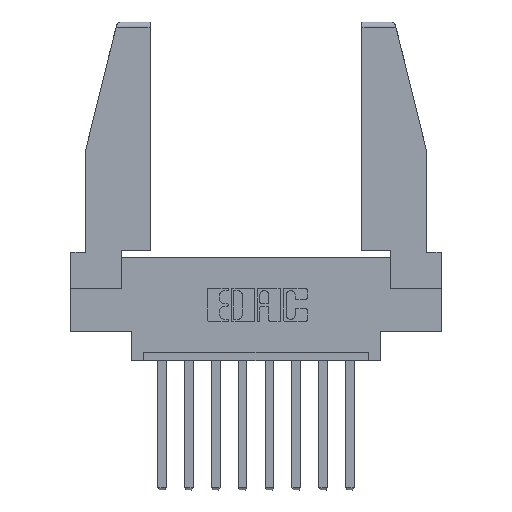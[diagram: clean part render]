
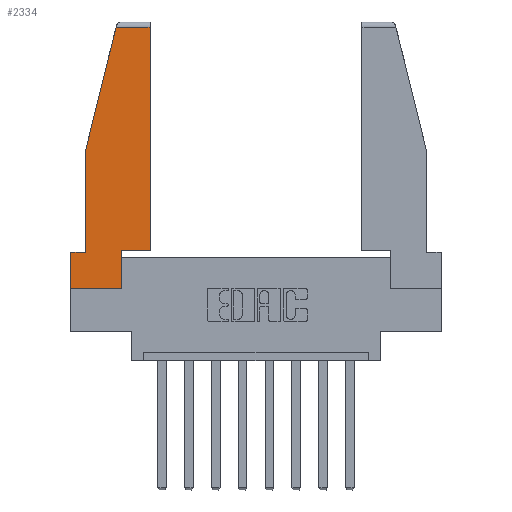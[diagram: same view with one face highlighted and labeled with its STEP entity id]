
A CAD part, top view. The second image highlights one B-rep face of the part: STEP entity #2334.
In plain terms, the highlighted planar face has unit normal (0, 0, 1).
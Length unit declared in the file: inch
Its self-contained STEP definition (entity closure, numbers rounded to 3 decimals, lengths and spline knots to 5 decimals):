
#14 = ORIENTED_EDGE ( 'NONE', *, *, #9014, .T. ) ;
#135 = CARTESIAN_POINT ( 'NONE',  ( 0., 0., 0. ) ) ;
#201 = ORIENTED_EDGE ( 'NONE', *, *, #7224, .T. ) ;
#439 = VERTEX_POINT ( 'NONE', #1502 ) ;
#717 = VERTEX_POINT ( 'NONE', #5867 ) ;
#740 = EDGE_CURVE ( 'NONE', #6335, #741, #3766, .T. ) ;
#741 = VERTEX_POINT ( 'NONE', #3374 ) ;
#911 = VECTOR ( 'NONE', #2036, 39.37008 ) ;
#1155 = DIRECTION ( 'NONE',  ( 1., 0., 0. ) ) ;
#1160 = EDGE_CURVE ( 'NONE', #439, #6132, #8548, .T. ) ;
#1394 = EDGE_CURVE ( 'NONE', #10571, #439, #8225, .T. ) ;
#1448 = CARTESIAN_POINT ( 'NONE',  ( 0.086, 0.21, 0. ) ) ;
#1502 = CARTESIAN_POINT ( 'NONE',  ( 0.297, 0., 0. ) ) ;
#1503 = DIRECTION ( 'NONE',  ( 1., 0., 0. ) ) ;
#1588 = DIRECTION ( 'NONE',  ( 0., 0., 1. ) ) ;
#1918 = VECTOR ( 'NONE', #4447, 39.37008 ) ;
#2019 = DIRECTION ( 'NONE',  ( 0., -1., 0. ) ) ;
#2036 = DIRECTION ( 'NONE',  ( -0.239, -0.971, 0. ) ) ;
#2334 = ADVANCED_FACE ( 'NONE', ( #7419 ), #7569, .T. ) ;
#2366 = VECTOR ( 'NONE', #6807, 39.37008 ) ;
#3278 = VECTOR ( 'NONE', #7551, 39.37008 ) ;
#3374 = CARTESIAN_POINT ( 'NONE',  ( 0., 0.21, 0. ) ) ;
#3446 = ORIENTED_EDGE ( 'NONE', *, *, #12394, .T. ) ;
#3766 = LINE ( 'NONE', #10461, #1918 ) ;
#4118 = VECTOR ( 'NONE', #6343, 39.37008 ) ;
#4447 = DIRECTION ( 'NONE',  ( -1., 0., 0. ) ) ;
#4508 = ORIENTED_EDGE ( 'NONE', *, *, #6766, .T. ) ;
#4559 = LINE ( 'NONE', #6667, #8242 ) ;
#4565 = VERTEX_POINT ( 'NONE', #8779 ) ;
#4630 = EDGE_CURVE ( 'NONE', #10523, #4565, #8130, .T. ) ;
#4658 = DIRECTION ( 'NONE',  ( 1., 0., 0. ) ) ;
#4681 = VECTOR ( 'NONE', #1155, 39.37008 ) ;
#5373 = CARTESIAN_POINT ( 'NONE',  ( 0., 0., 0. ) ) ;
#5867 = CARTESIAN_POINT ( 'NONE',  ( 0.086, 0.8, 0. ) ) ;
#6132 = VERTEX_POINT ( 'NONE', #8442 ) ;
#6335 = VERTEX_POINT ( 'NONE', #1448 ) ;
#6343 = DIRECTION ( 'NONE',  ( -1., 0., 0. ) ) ;
#6373 = ORIENTED_EDGE ( 'NONE', *, *, #740, .T. ) ;
#6431 = ORIENTED_EDGE ( 'NONE', *, *, #9696, .T. ) ;
#6667 = CARTESIAN_POINT ( 'NONE',  ( 0.297, 0.223, 0. ) ) ;
#6766 = EDGE_CURVE ( 'NONE', #12719, #10523, #12225, .T. ) ;
#6783 = LINE ( 'NONE', #10867, #911 ) ;
#6807 = DIRECTION ( 'NONE',  ( 0., 1., 0. ) ) ;
#7224 = EDGE_CURVE ( 'NONE', #717, #6335, #12501, .T. ) ;
#7419 = FACE_OUTER_BOUND ( 'NONE', #7625, .T. ) ;
#7424 = CARTESIAN_POINT ( 'NONE',  ( 0., 1.52, 0. ) ) ;
#7551 = DIRECTION ( 'NONE',  ( 0., 1., 0. ) ) ;
#7569 = PLANE ( 'NONE',  #9870 ) ;
#7625 = EDGE_LOOP ( 'NONE', ( #4508, #8497, #14, #201, #6373, #6431, #11164, #10356, #3446 ) ) ;
#7765 = CARTESIAN_POINT ( 'NONE',  ( 0.461, 0.223, 0. ) ) ;
#8130 = LINE ( 'NONE', #7424, #4118 ) ;
#8224 = DIRECTION ( 'NONE',  ( 0., -1., 0. ) ) ;
#8225 = LINE ( 'NONE', #135, #4681 ) ;
#8242 = VECTOR ( 'NONE', #4658, 39.37008 ) ;
#8442 = CARTESIAN_POINT ( 'NONE',  ( 0.297, 0.223, 0. ) ) ;
#8497 = ORIENTED_EDGE ( 'NONE', *, *, #4630, .T. ) ;
#8548 = LINE ( 'NONE', #9742, #3278 ) ;
#8779 = CARTESIAN_POINT ( 'NONE',  ( 0.2636, 1.52, 0. ) ) ;
#9014 = EDGE_CURVE ( 'NONE', #4565, #717, #6783, .T. ) ;
#9696 = EDGE_CURVE ( 'NONE', #741, #10571, #10022, .T. ) ;
#9742 = CARTESIAN_POINT ( 'NONE',  ( 0.297, 0., 0. ) ) ;
#9866 = VECTOR ( 'NONE', #8224, 39.37008 ) ;
#9870 = AXIS2_PLACEMENT_3D ( 'NONE', #10474, #1588, #1503 ) ;
#10022 = LINE ( 'NONE', #11097, #9866 ) ;
#10324 = CARTESIAN_POINT ( 'NONE',  ( 0.461, 1.52, 0. ) ) ;
#10356 = ORIENTED_EDGE ( 'NONE', *, *, #1160, .T. ) ;
#10461 = CARTESIAN_POINT ( 'NONE',  ( 0., 0.21, 0. ) ) ;
#10474 = CARTESIAN_POINT ( 'NONE',  ( 0., 0., 0. ) ) ;
#10523 = VERTEX_POINT ( 'NONE', #10324 ) ;
#10571 = VERTEX_POINT ( 'NONE', #5373 ) ;
#10797 = CARTESIAN_POINT ( 'NONE',  ( 0.461, 0.223, 0. ) ) ;
#10867 = CARTESIAN_POINT ( 'NONE',  ( 0.271, 1.55, 0. ) ) ;
#10932 = CARTESIAN_POINT ( 'NONE',  ( 0.086, 0.8, 0. ) ) ;
#11097 = CARTESIAN_POINT ( 'NONE',  ( 0., 0.21, 0. ) ) ;
#11164 = ORIENTED_EDGE ( 'NONE', *, *, #1394, .T. ) ;
#11903 = VECTOR ( 'NONE', #2019, 39.37008 ) ;
#12225 = LINE ( 'NONE', #7765, #2366 ) ;
#12394 = EDGE_CURVE ( 'NONE', #6132, #12719, #4559, .T. ) ;
#12501 = LINE ( 'NONE', #10932, #11903 ) ;
#12719 = VERTEX_POINT ( 'NONE', #10797 ) ;
